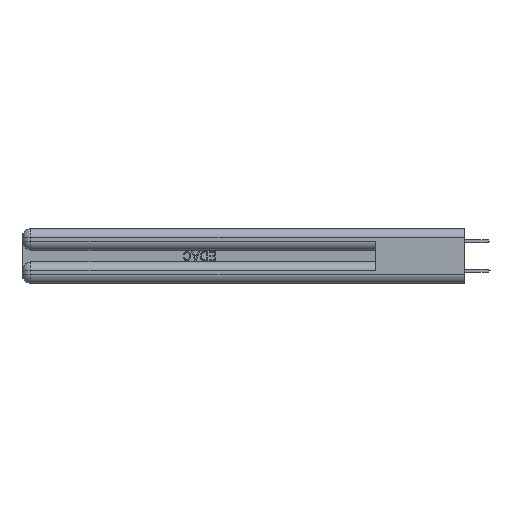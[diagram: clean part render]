
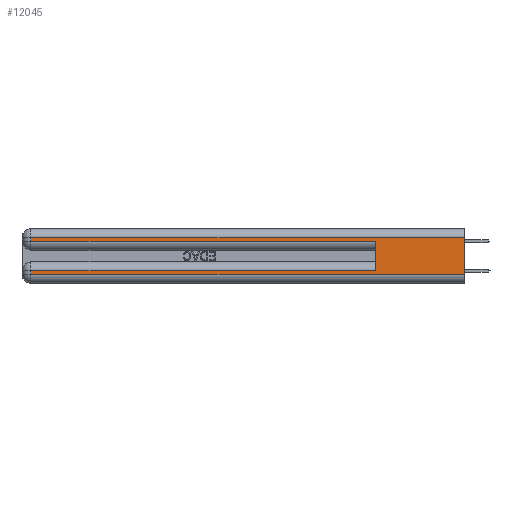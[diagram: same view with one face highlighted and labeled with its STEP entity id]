
A CAD part, left-side view. The second image highlights one B-rep face of the part: STEP entity #12045.
In plain terms, the highlighted planar face has unit normal (-1, 0, 0).
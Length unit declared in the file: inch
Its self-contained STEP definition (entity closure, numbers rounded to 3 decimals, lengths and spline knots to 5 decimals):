
#1052 = ORIENTED_EDGE ( 'NONE', *, *, #20474, .T. ) ;
#1414 = CARTESIAN_POINT ( 'NONE',  ( 0., 0., 0.085 ) ) ;
#1427 = DIRECTION ( 'NONE',  ( 0., 1., 0. ) ) ;
#1461 = CARTESIAN_POINT ( 'NONE',  ( 0., 2.94, 0.37 ) ) ;
#4307 = CARTESIAN_POINT ( 'NONE',  ( 0., 2.94, 0.37 ) ) ;
#4371 = EDGE_LOOP ( 'NONE', ( #45817, #32433, #24994, #1052, #13610, #7533, #22347, #12905 ) ) ;
#4444 = LINE ( 'NONE', #47321, #12036 ) ;
#5546 = VECTOR ( 'NONE', #23750, 39.37008 ) ;
#5920 = EDGE_CURVE ( 'NONE', #9655, #25605, #8887, .T. ) ;
#6066 = VERTEX_POINT ( 'NONE', #38857 ) ;
#6398 = CARTESIAN_POINT ( 'NONE',  ( 0., 0.6, 0.285 ) ) ;
#6544 = LINE ( 'NONE', #12069, #33549 ) ;
#7252 = AXIS2_PLACEMENT_3D ( 'NONE', #33884, #37494, #15693 ) ;
#7517 = DIRECTION ( 'NONE',  ( 0., 0., -1. ) ) ;
#7533 = ORIENTED_EDGE ( 'NONE', *, *, #34009, .T. ) ;
#8179 = PLANE ( 'NONE',  #7252 ) ;
#8887 = LINE ( 'NONE', #20016, #35857 ) ;
#9196 = CARTESIAN_POINT ( 'NONE',  ( 0., 0., 0.31 ) ) ;
#9594 = CARTESIAN_POINT ( 'NONE',  ( 0., 0., 0.06 ) ) ;
#9655 = VERTEX_POINT ( 'NONE', #9196 ) ;
#9829 = FACE_OUTER_BOUND ( 'NONE', #4371, .T. ) ;
#11149 = VECTOR ( 'NONE', #28729, 39.37008 ) ;
#11381 = VERTEX_POINT ( 'NONE', #37878 ) ;
#12036 = VECTOR ( 'NONE', #7517, 39.37008 ) ;
#12045 = ADVANCED_FACE ( 'NONE', ( #9829 ), #8179, .F. ) ;
#12069 = CARTESIAN_POINT ( 'NONE',  ( 0., 0., 0.06 ) ) ;
#12704 = VERTEX_POINT ( 'NONE', #29430 ) ;
#12905 = ORIENTED_EDGE ( 'NONE', *, *, #40246, .T. ) ;
#13610 = ORIENTED_EDGE ( 'NONE', *, *, #35749, .F. ) ;
#13875 = VECTOR ( 'NONE', #16267, 39.37008 ) ;
#14027 = EDGE_CURVE ( 'NONE', #9655, #42207, #4444, .T. ) ;
#15693 = DIRECTION ( 'NONE',  ( 0., 0., -1. ) ) ;
#16267 = DIRECTION ( 'NONE',  ( 0., 1., 0. ) ) ;
#18214 = CARTESIAN_POINT ( 'NONE',  ( 0., 0.6, 0.085 ) ) ;
#18269 = VERTEX_POINT ( 'NONE', #18214 ) ;
#20016 = CARTESIAN_POINT ( 'NONE',  ( 0., 0., 0.31 ) ) ;
#20474 = EDGE_CURVE ( 'NONE', #12704, #22524, #40293, .T. ) ;
#21356 = CARTESIAN_POINT ( 'NONE',  ( 0., 0., 0.285 ) ) ;
#22347 = ORIENTED_EDGE ( 'NONE', *, *, #27523, .T. ) ;
#22524 = VERTEX_POINT ( 'NONE', #6398 ) ;
#23270 = DIRECTION ( 'NONE',  ( 0., -1., 0. ) ) ;
#23750 = DIRECTION ( 'NONE',  ( 0., 0., -1. ) ) ;
#24866 = LINE ( 'NONE', #1414, #13875 ) ;
#24994 = ORIENTED_EDGE ( 'NONE', *, *, #46640, .T. ) ;
#25605 = VERTEX_POINT ( 'NONE', #44841 ) ;
#27523 = EDGE_CURVE ( 'NONE', #11381, #6066, #44413, .T. ) ;
#28729 = DIRECTION ( 'NONE',  ( 0., -1., 0. ) ) ;
#29430 = CARTESIAN_POINT ( 'NONE',  ( 0., 2.94, 0.285 ) ) ;
#29501 = VECTOR ( 'NONE', #44590, 39.37008 ) ;
#32114 = VECTOR ( 'NONE', #46034, 39.37008 ) ;
#32433 = ORIENTED_EDGE ( 'NONE', *, *, #5920, .T. ) ;
#33549 = VECTOR ( 'NONE', #23270, 39.37008 ) ;
#33884 = CARTESIAN_POINT ( 'NONE',  ( 0., 0., 0.37 ) ) ;
#34009 = EDGE_CURVE ( 'NONE', #18269, #11381, #24866, .T. ) ;
#35749 = EDGE_CURVE ( 'NONE', #18269, #22524, #41657, .T. ) ;
#35857 = VECTOR ( 'NONE', #1427, 39.37008 ) ;
#36228 = CARTESIAN_POINT ( 'NONE',  ( 0., 0.6, 0.145 ) ) ;
#37494 = DIRECTION ( 'NONE',  ( 1., 0., 0. ) ) ;
#37878 = CARTESIAN_POINT ( 'NONE',  ( 0., 2.94, 0.085 ) ) ;
#38857 = CARTESIAN_POINT ( 'NONE',  ( 0., 2.94, 0.06 ) ) ;
#39041 = LINE ( 'NONE', #4307, #29501 ) ;
#40246 = EDGE_CURVE ( 'NONE', #6066, #42207, #6544, .T. ) ;
#40293 = LINE ( 'NONE', #21356, #11149 ) ;
#41657 = LINE ( 'NONE', #36228, #32114 ) ;
#42207 = VERTEX_POINT ( 'NONE', #9594 ) ;
#44413 = LINE ( 'NONE', #1461, #5546 ) ;
#44590 = DIRECTION ( 'NONE',  ( 0., 0., -1. ) ) ;
#44841 = CARTESIAN_POINT ( 'NONE',  ( 0., 2.94, 0.31 ) ) ;
#45817 = ORIENTED_EDGE ( 'NONE', *, *, #14027, .F. ) ;
#46034 = DIRECTION ( 'NONE',  ( 0., 0., 1. ) ) ;
#46640 = EDGE_CURVE ( 'NONE', #25605, #12704, #39041, .T. ) ;
#47321 = CARTESIAN_POINT ( 'NONE',  ( 0., 0., 0.37 ) ) ;
